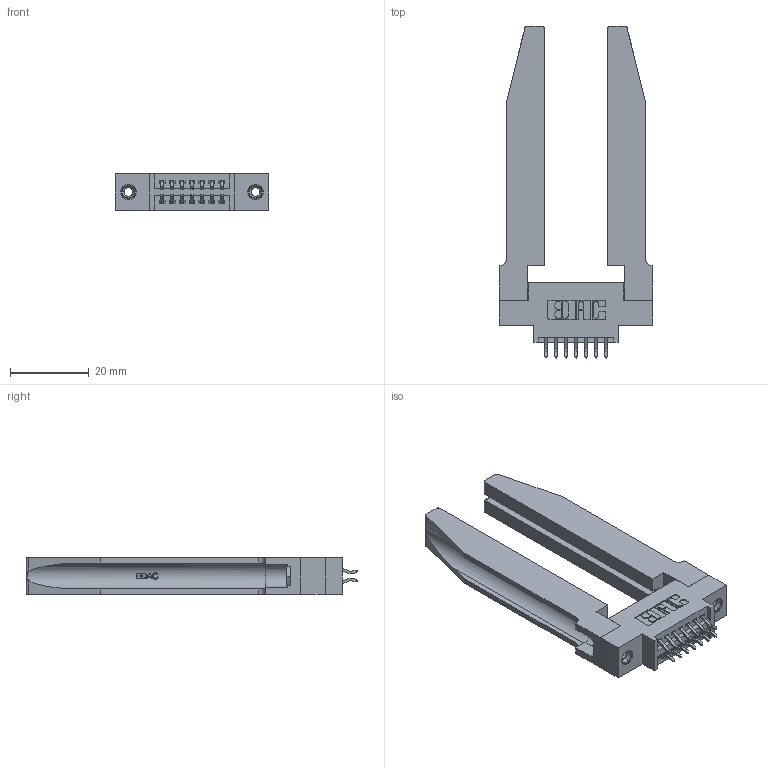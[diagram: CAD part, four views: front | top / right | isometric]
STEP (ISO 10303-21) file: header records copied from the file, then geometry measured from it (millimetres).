
FILE_DESCRIPTION (( 'STEP AP203' ), '1' );
FILE_NAME ('395-014-556-878.STEP', '2019-10-15T16:49:28', ( '' ), ( '' ), 'SwSTEP 2.0', 'SolidWorks 2016', '' );
FILE_SCHEMA (( 'CONFIG_CONTROL_DESIGN' ));
Length unit declared in the file: inch
Products named in the file (5): 395-014-556-878; 345 Part_0.170 Offset - 0.156 Dia-TH; 345-292-001_556 Tail; 345-250-001_345-250-001-102; 345-220-078_345-220-078
Assembly tree (19 placements, depth 2):
  395-014-556-878
    345 Part_0.170 Offset - 0.156 Dia-TH
    345-292-001_556 Tail  x14
    345-250-001_345-250-001-102  x2
    345-220-078_345-220-078  x2
Bounding box: 39.01 x 84.51 x 9.4 mm (x, y, z)
Volume: 11121.5 mm3; surface area: 11245.2 mm2
Topology: 19 solids, 19 shells, 1148 faces, 3299 edges, 2170 vertices
Faces by surface type: plane 744, cylinder 352, bspline 36, cone 12, torus 4
Entity records: 15296 total; most frequent: CARTESIAN_POINT 3531, ORIENTED_EDGE 2350, DIRECTION 2137, EDGE_CURVE 1175, LINE 913, VECTOR 913, VERTEX_POINT 776, AXIS2_PLACEMENT_3D 612
